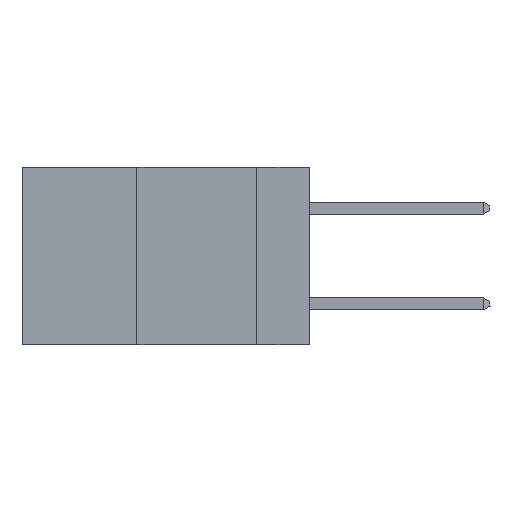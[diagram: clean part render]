
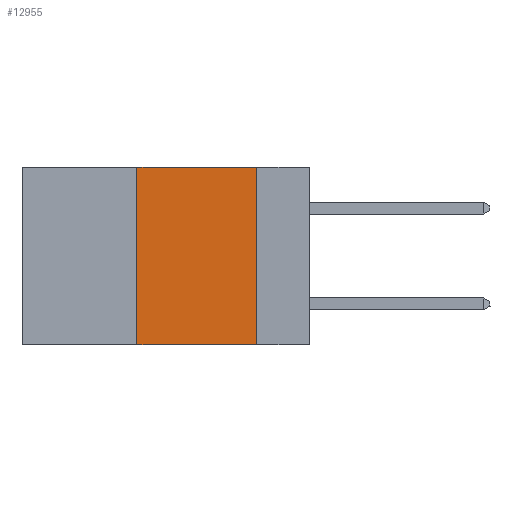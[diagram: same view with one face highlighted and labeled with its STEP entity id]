
A CAD part, left-side view. The second image highlights one B-rep face of the part: STEP entity #12955.
In plain terms, the highlighted planar face has unit normal (-1, 0, 0).
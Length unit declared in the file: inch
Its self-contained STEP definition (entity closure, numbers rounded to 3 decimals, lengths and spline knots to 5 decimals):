
#1145 = CARTESIAN_POINT ( 'NONE',  ( 0., 0.6, 0. ) ) ;
#1969 = ORIENTED_EDGE ( 'NONE', *, *, #15632, .T. ) ;
#2292 = PLANE ( 'NONE',  #12667 ) ;
#2474 = CARTESIAN_POINT ( 'NONE',  ( 0., 0.11, 0. ) ) ;
#3460 = ORIENTED_EDGE ( 'NONE', *, *, #29803, .F. ) ;
#5526 = ORIENTED_EDGE ( 'NONE', *, *, #15063, .F. ) ;
#6068 = DIRECTION ( 'NONE',  ( 0., 0., 1. ) ) ;
#8279 = VECTOR ( 'NONE', #10510, 39.37008 ) ;
#10510 = DIRECTION ( 'NONE',  ( 0., -1., 0. ) ) ;
#11655 = DIRECTION ( 'NONE',  ( 1., 0., 0. ) ) ;
#12667 = AXIS2_PLACEMENT_3D ( 'NONE', #23314, #11655, #18868 ) ;
#12955 = ADVANCED_FACE ( 'NONE', ( #21173 ), #2292, .F. ) ;
#13875 = CARTESIAN_POINT ( 'NONE',  ( 0., 0.36, 0. ) ) ;
#13965 = EDGE_LOOP ( 'NONE', ( #16828, #5526, #3460, #1969 ) ) ;
#14172 = CARTESIAN_POINT ( 'NONE',  ( 0., 0.11, 0. ) ) ;
#15063 = EDGE_CURVE ( 'NONE', #24692, #21527, #22182, .T. ) ;
#15632 = EDGE_CURVE ( 'NONE', #24691, #25971, #29769, .T. ) ;
#16828 = ORIENTED_EDGE ( 'NONE', *, *, #23426, .F. ) ;
#18868 = DIRECTION ( 'NONE',  ( 0., 0., -1. ) ) ;
#19896 = LINE ( 'NONE', #20334, #27241 ) ;
#20334 = CARTESIAN_POINT ( 'NONE',  ( 0., 0.36, 0. ) ) ;
#20785 = CARTESIAN_POINT ( 'NONE',  ( 0., 0.36, -0.37 ) ) ;
#21041 = VECTOR ( 'NONE', #23342, 39.37008 ) ;
#21173 = FACE_OUTER_BOUND ( 'NONE', #13965, .T. ) ;
#21201 = LINE ( 'NONE', #2474, #24725 ) ;
#21527 = VERTEX_POINT ( 'NONE', #14172 ) ;
#22182 = LINE ( 'NONE', #1145, #8279 ) ;
#23033 = CARTESIAN_POINT ( 'NONE',  ( 0., 0.6, -0.37 ) ) ;
#23314 = CARTESIAN_POINT ( 'NONE',  ( 0., 0.6, 0. ) ) ;
#23342 = DIRECTION ( 'NONE',  ( 0., -1., 0. ) ) ;
#23426 = EDGE_CURVE ( 'NONE', #21527, #25971, #21201, .T. ) ;
#24691 = VERTEX_POINT ( 'NONE', #20785 ) ;
#24692 = VERTEX_POINT ( 'NONE', #13875 ) ;
#24725 = VECTOR ( 'NONE', #25943, 39.37008 ) ;
#25943 = DIRECTION ( 'NONE',  ( 0., 0., -1. ) ) ;
#25971 = VERTEX_POINT ( 'NONE', #27142 ) ;
#27142 = CARTESIAN_POINT ( 'NONE',  ( 0., 0.11, -0.37 ) ) ;
#27241 = VECTOR ( 'NONE', #6068, 39.37008 ) ;
#29769 = LINE ( 'NONE', #23033, #21041 ) ;
#29803 = EDGE_CURVE ( 'NONE', #24691, #24692, #19896, .T. ) ;
